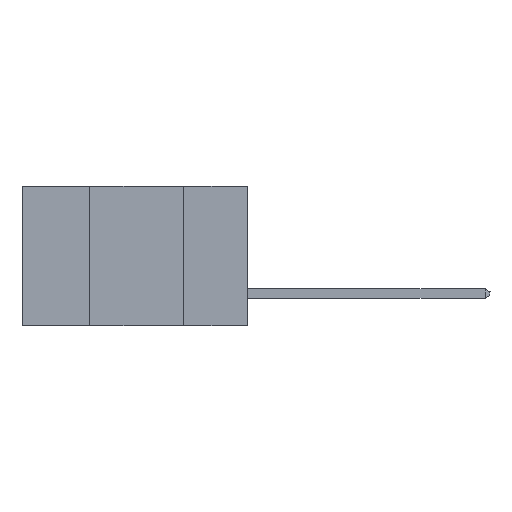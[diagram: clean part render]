
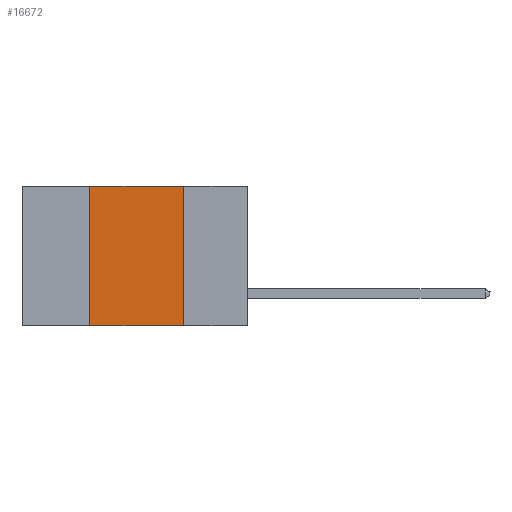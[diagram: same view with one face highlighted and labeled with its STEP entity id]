
A CAD part, left-side view. The second image highlights one B-rep face of the part: STEP entity #16672.
In plain terms, the highlighted planar face has unit normal (-1, 0, 0).
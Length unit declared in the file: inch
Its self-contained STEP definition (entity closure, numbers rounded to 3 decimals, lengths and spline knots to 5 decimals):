
#439 = PLANE ( 'NONE',  #20132 ) ;
#1149 = DIRECTION ( 'NONE',  ( 0., -1., 0. ) ) ;
#1327 = ORIENTED_EDGE ( 'NONE', *, *, #19520, .F. ) ;
#2687 = VECTOR ( 'NONE', #1149, 39.37008 ) ;
#3085 = VERTEX_POINT ( 'NONE', #7859 ) ;
#3754 = VERTEX_POINT ( 'NONE', #15036 ) ;
#3843 = EDGE_CURVE ( 'NONE', #13645, #3085, #19456, .T. ) ;
#6753 = ORIENTED_EDGE ( 'NONE', *, *, #22497, .F. ) ;
#7185 = CARTESIAN_POINT ( 'NONE',  ( 0., 0.6, 0. ) ) ;
#7532 = DIRECTION ( 'NONE',  ( 1., 0., 0. ) ) ;
#7740 = EDGE_LOOP ( 'NONE', ( #1327, #6753, #18770, #20558 ) ) ;
#7859 = CARTESIAN_POINT ( 'NONE',  ( 0., 0.42, 0. ) ) ;
#7993 = LINE ( 'NONE', #16924, #8408 ) ;
#8367 = VECTOR ( 'NONE', #14502, 39.37008 ) ;
#8408 = VECTOR ( 'NONE', #11575, 39.37008 ) ;
#9855 = CARTESIAN_POINT ( 'NONE',  ( 0., 0.6, -0.37 ) ) ;
#10500 = VECTOR ( 'NONE', #20837, 39.37008 ) ;
#10866 = DIRECTION ( 'NONE',  ( 0., 0., -1. ) ) ;
#11077 = CARTESIAN_POINT ( 'NONE',  ( 0., 0.17, 0. ) ) ;
#11575 = DIRECTION ( 'NONE',  ( 0., -1., 0. ) ) ;
#12850 = FACE_OUTER_BOUND ( 'NONE', #7740, .T. ) ;
#13645 = VERTEX_POINT ( 'NONE', #22803 ) ;
#14502 = DIRECTION ( 'NONE',  ( 0., 0., -1. ) ) ;
#15036 = CARTESIAN_POINT ( 'NONE',  ( 0., 0.17, -0.37 ) ) ;
#16359 = EDGE_CURVE ( 'NONE', #13645, #3754, #16937, .T. ) ;
#16360 = CARTESIAN_POINT ( 'NONE',  ( 0., 0.17, -0.37 ) ) ;
#16672 = ADVANCED_FACE ( 'NONE', ( #12850 ), #439, .F. ) ;
#16924 = CARTESIAN_POINT ( 'NONE',  ( 0., 0.6, 0. ) ) ;
#16937 = LINE ( 'NONE', #9855, #2687 ) ;
#18770 = ORIENTED_EDGE ( 'NONE', *, *, #3843, .F. ) ;
#19342 = CARTESIAN_POINT ( 'NONE',  ( 0., 0.42, -0.37 ) ) ;
#19456 = LINE ( 'NONE', #19342, #10500 ) ;
#19520 = EDGE_CURVE ( 'NONE', #19944, #3754, #19968, .T. ) ;
#19944 = VERTEX_POINT ( 'NONE', #11077 ) ;
#19968 = LINE ( 'NONE', #16360, #8367 ) ;
#20132 = AXIS2_PLACEMENT_3D ( 'NONE', #7185, #7532, #10866 ) ;
#20558 = ORIENTED_EDGE ( 'NONE', *, *, #16359, .T. ) ;
#20837 = DIRECTION ( 'NONE',  ( 0., 0., 1. ) ) ;
#22497 = EDGE_CURVE ( 'NONE', #3085, #19944, #7993, .T. ) ;
#22803 = CARTESIAN_POINT ( 'NONE',  ( 0., 0.42, -0.37 ) ) ;
